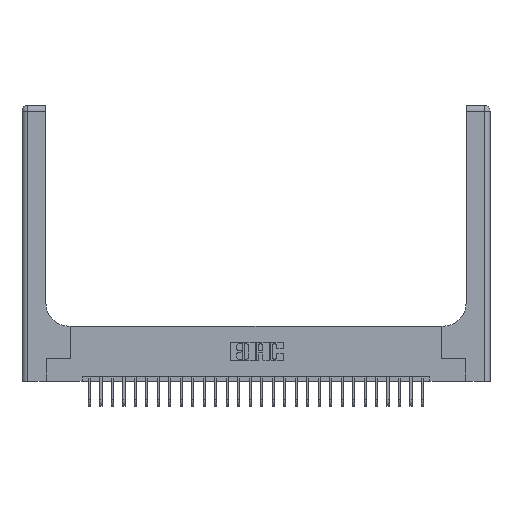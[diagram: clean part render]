
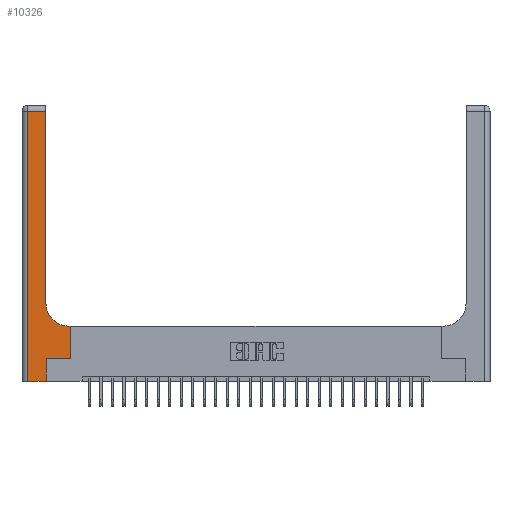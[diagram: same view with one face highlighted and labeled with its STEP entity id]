
A CAD part, top view. The second image highlights one B-rep face of the part: STEP entity #10326.
In plain terms, the highlighted planar face has unit normal (0, 0, 1).
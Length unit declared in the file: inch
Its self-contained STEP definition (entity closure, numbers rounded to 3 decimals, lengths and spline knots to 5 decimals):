
#134 = AXIS2_PLACEMENT_3D ( 'NONE', #1234, #15047, #3226 ) ;
#246 = ORIENTED_EDGE ( 'NONE', *, *, #5648, .T. ) ;
#314 = DIRECTION ( 'NONE',  ( 1., 0., 0. ) ) ;
#447 = VERTEX_POINT ( 'NONE', #10479 ) ;
#757 = DIRECTION ( 'NONE',  ( -1., 0., 0. ) ) ;
#865 = CARTESIAN_POINT ( 'NONE',  ( 0.26, 3., 0.37 ) ) ;
#1234 = CARTESIAN_POINT ( 'NONE',  ( 0.51, 0.85, 0.37 ) ) ;
#1252 = ORIENTED_EDGE ( 'NONE', *, *, #15201, .T. ) ;
#2383 = VERTEX_POINT ( 'NONE', #9267 ) ;
#2438 = CARTESIAN_POINT ( 'NONE',  ( 0.265, 0.25, 0.37 ) ) ;
#2659 = CARTESIAN_POINT ( 'NONE',  ( 0.265, 0., 0.37 ) ) ;
#3051 = DIRECTION ( 'NONE',  ( 0., -1., 0. ) ) ;
#3226 = DIRECTION ( 'NONE',  ( 1., 0., 0. ) ) ;
#3772 = CARTESIAN_POINT ( 'NONE',  ( 0.26, 0.6, 0.37 ) ) ;
#4023 = VERTEX_POINT ( 'NONE', #17204 ) ;
#4054 = VERTEX_POINT ( 'NONE', #9442 ) ;
#4707 = ORIENTED_EDGE ( 'NONE', *, *, #24802, .T. ) ;
#4733 = CARTESIAN_POINT ( 'NONE',  ( 0., 2.94, 0.37 ) ) ;
#5022 = VERTEX_POINT ( 'NONE', #13832 ) ;
#5315 = EDGE_CURVE ( 'NONE', #447, #21459, #21530, .T. ) ;
#5648 = EDGE_CURVE ( 'NONE', #4054, #23220, #8886, .T. ) ;
#5731 = VECTOR ( 'NONE', #314, 39.37008 ) ;
#5902 = VECTOR ( 'NONE', #18481, 39.37008 ) ;
#6160 = ORIENTED_EDGE ( 'NONE', *, *, #10331, .T. ) ;
#6554 = ORIENTED_EDGE ( 'NONE', *, *, #21245, .T. ) ;
#8886 = LINE ( 'NONE', #3772, #9489 ) ;
#9267 = CARTESIAN_POINT ( 'NONE',  ( 0.528, 0.25, 0.37 ) ) ;
#9323 = CARTESIAN_POINT ( 'NONE',  ( 0.528, 0.25, 0.37 ) ) ;
#9442 = CARTESIAN_POINT ( 'NONE',  ( 0.528, 0.6, 0.37 ) ) ;
#9489 = VECTOR ( 'NONE', #19512, 39.37008 ) ;
#9693 = VECTOR ( 'NONE', #3051, 39.37008 ) ;
#9909 = EDGE_CURVE ( 'NONE', #21796, #5022, #15192, .T. ) ;
#10142 = CARTESIAN_POINT ( 'NONE',  ( 0.265, 0.25, 0.37 ) ) ;
#10326 = ADVANCED_FACE ( 'NONE', ( #15782 ), #10565, .F. ) ;
#10331 = EDGE_CURVE ( 'NONE', #21459, #4023, #10502, .T. ) ;
#10479 = CARTESIAN_POINT ( 'NONE',  ( 0.26, 0.85, 0.37 ) ) ;
#10502 = LINE ( 'NONE', #4733, #5902 ) ;
#10565 = PLANE ( 'NONE',  #10991 ) ;
#10635 = CARTESIAN_POINT ( 'NONE',  ( 0.26, 2.94, 0.37 ) ) ;
#10991 = AXIS2_PLACEMENT_3D ( 'NONE', #22395, #12590, #757 ) ;
#11238 = DIRECTION ( 'NONE',  ( 1., 0., 0. ) ) ;
#12590 = DIRECTION ( 'NONE',  ( 0., 0., -1. ) ) ;
#13239 = CARTESIAN_POINT ( 'NONE',  ( 0., 0., 0.37 ) ) ;
#13353 = EDGE_CURVE ( 'NONE', #2383, #4054, #15942, .T. ) ;
#13832 = CARTESIAN_POINT ( 'NONE',  ( 0.265, 0., 0.37 ) ) ;
#14613 = ORIENTED_EDGE ( 'NONE', *, *, #5315, .T. ) ;
#14681 = DIRECTION ( 'NONE',  ( 0., 1., 0. ) ) ;
#14834 = ORIENTED_EDGE ( 'NONE', *, *, #23412, .T. ) ;
#14992 = VERTEX_POINT ( 'NONE', #2438 ) ;
#15047 = DIRECTION ( 'NONE',  ( 0., 0., -1. ) ) ;
#15157 = CARTESIAN_POINT ( 'NONE',  ( 0.06, 0., 0.37 ) ) ;
#15192 = LINE ( 'NONE', #13239, #19763 ) ;
#15201 = EDGE_CURVE ( 'NONE', #4023, #21796, #25396, .T. ) ;
#15619 = LINE ( 'NONE', #10142, #5731 ) ;
#15782 = FACE_OUTER_BOUND ( 'NONE', #18838, .T. ) ;
#15942 = LINE ( 'NONE', #9323, #20543 ) ;
#15954 = CARTESIAN_POINT ( 'NONE',  ( 0.51, 0.6, 0.37 ) ) ;
#16839 = CARTESIAN_POINT ( 'NONE',  ( 0.06, 3., 0.37 ) ) ;
#17204 = CARTESIAN_POINT ( 'NONE',  ( 0.06, 2.94, 0.37 ) ) ;
#17248 = DIRECTION ( 'NONE',  ( 0., 1., 0. ) ) ;
#18481 = DIRECTION ( 'NONE',  ( -1., 0., 0. ) ) ;
#18614 = CIRCLE ( 'NONE', #134, 0.25 ) ;
#18838 = EDGE_LOOP ( 'NONE', ( #14613, #6160, #1252, #20249, #14834, #6554, #22755, #246, #4707 ) ) ;
#19321 = VECTOR ( 'NONE', #24354, 39.37008 ) ;
#19512 = DIRECTION ( 'NONE',  ( -1., 0., 0. ) ) ;
#19763 = VECTOR ( 'NONE', #11238, 39.37008 ) ;
#19927 = LINE ( 'NONE', #2659, #19321 ) ;
#20249 = ORIENTED_EDGE ( 'NONE', *, *, #9909, .T. ) ;
#20543 = VECTOR ( 'NONE', #17248, 39.37008 ) ;
#20919 = VECTOR ( 'NONE', #14681, 39.37008 ) ;
#21245 = EDGE_CURVE ( 'NONE', #14992, #2383, #15619, .T. ) ;
#21459 = VERTEX_POINT ( 'NONE', #10635 ) ;
#21530 = LINE ( 'NONE', #865, #20919 ) ;
#21796 = VERTEX_POINT ( 'NONE', #15157 ) ;
#22395 = CARTESIAN_POINT ( 'NONE',  ( 0., 3., 0.37 ) ) ;
#22755 = ORIENTED_EDGE ( 'NONE', *, *, #13353, .T. ) ;
#23220 = VERTEX_POINT ( 'NONE', #15954 ) ;
#23412 = EDGE_CURVE ( 'NONE', #5022, #14992, #19927, .T. ) ;
#24354 = DIRECTION ( 'NONE',  ( 0., 1., 0. ) ) ;
#24802 = EDGE_CURVE ( 'NONE', #23220, #447, #18614, .T. ) ;
#25396 = LINE ( 'NONE', #16839, #9693 ) ;
